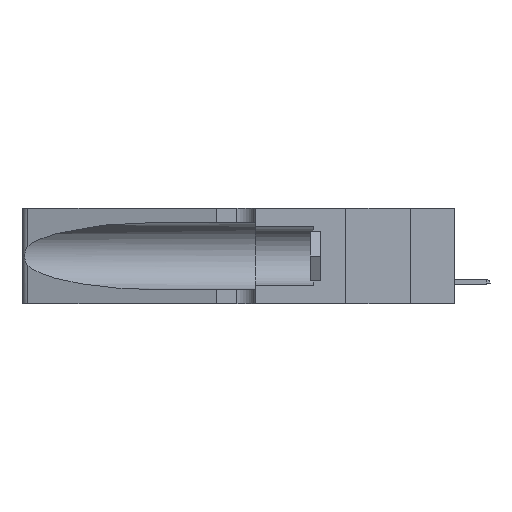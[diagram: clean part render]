
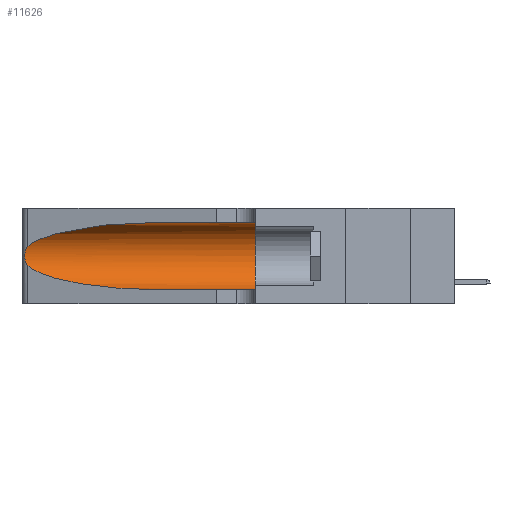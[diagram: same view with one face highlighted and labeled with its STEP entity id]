
A CAD part, left-side view. The second image highlights one B-rep face of the part: STEP entity #11626.
In plain terms, the highlighted cylindrical face has radius 3.308 mm (diameter 6.617 mm), a partial arc.
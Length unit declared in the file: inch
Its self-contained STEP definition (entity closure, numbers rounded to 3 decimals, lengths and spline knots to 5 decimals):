
#151 = VERTEX_POINT ( 'NONE', #3501 ) ;
#190 = DIRECTION ( 'NONE',  ( 0., -1., 0. ) ) ;
#1014 = CARTESIAN_POINT ( 'NONE',  ( 0.18966, 0.96281, 0.31525 ) ) ;
#1051 = CARTESIAN_POINT ( 'NONE',  ( 0.25555, 1.22993, 0.14849 ) ) ;
#1424 = CARTESIAN_POINT ( 'NONE',  ( 0.25787, 1.23484, 0.2124 ) ) ;
#2444 = CARTESIAN_POINT ( 'NONE',  ( 0.25487, 1.22718, 0.14631 ) ) ;
#2725 = VECTOR ( 'NONE', #190, 39.37008 ) ;
#3114 = CARTESIAN_POINT ( 'NONE',  ( 0.26075, 1.23896, 0.178 ) ) ;
#3232 = EDGE_CURVE ( 'NONE', #11113, #3688, #13673, .T. ) ;
#3237 = CARTESIAN_POINT ( 'NONE',  ( 0.26017, 1.23833, 0.17102 ) ) ;
#3501 = CARTESIAN_POINT ( 'NONE',  ( 0.1305, 0.72297, 0.31525 ) ) ;
#3611 = CARTESIAN_POINT ( 'NONE',  ( 0.25487, 1.22718, 0.22369 ) ) ;
#3688 = VERTEX_POINT ( 'NONE', #20393 ) ;
#4425 = B_SPLINE_CURVE_WITH_KNOTS ( 'NONE', 3,
 ( #3611, #5035, #24496, #1424, #21156, #20654, #14872, #3114, #3237, #16923, #13206, #11416, #1051, #5421 ),
 .UNSPECIFIED., .F., .F.,
 ( 4, 2, 2, 2, 2, 2, 4 ),
 ( 0., 0.00027, 0.00053, 0.00107, 0.0016, 0.00187, 0.00214 ),
 .UNSPECIFIED. ) ;
#4504 = CARTESIAN_POINT ( 'NONE',  ( 0.25487, 1.22718, 0.22369 ) ) ;
#4877 = CARTESIAN_POINT ( 'NONE',  ( 0.1305, 0.35, 0.31525 ) ) ;
#5028 = EDGE_CURVE ( 'NONE', #7660, #12169, #4425, .T. ) ;
#5035 = CARTESIAN_POINT ( 'NONE',  ( 0.25555, 1.22994, 0.2215 ) ) ;
#5104 = EDGE_CURVE ( 'NONE', #151, #11113, #6177, .T. ) ;
#5421 = CARTESIAN_POINT ( 'NONE',  ( 0.25487, 1.22718, 0.14631 ) ) ;
#5674 = ORIENTED_EDGE ( 'NONE', *, *, #12125, .T. ) ;
#6177 = LINE ( 'NONE', #19471, #2725 ) ;
#6364 = DIRECTION ( 'NONE',  ( 0., 0., 1. ) ) ;
#6689 =( BOUNDED_CURVE ( )  B_SPLINE_CURVE ( 3, ( #16148, #14227, #23962, #22038 ),
 .UNSPECIFIED., .F., .F. ) 
 B_SPLINE_CURVE_WITH_KNOTS ( ( 4, 4 ),
 ( 3.44316, 4.71239 ),
 .UNSPECIFIED. ) 
 CURVE ( )  GEOMETRIC_REPRESENTATION_ITEM ( )  RATIONAL_B_SPLINE_CURVE ( ( 1., 0.87, 0.87, 1. ) ) 
 REPRESENTATION_ITEM ( '' )  );
#6929 = CARTESIAN_POINT ( 'NONE',  ( 0.1305, 0.72297, 0.31525 ) ) ;
#7660 = VERTEX_POINT ( 'NONE', #21090 ) ;
#7761 = CARTESIAN_POINT ( 'NONE',  ( 0.1305, 0.72297, 0.05475 ) ) ;
#8336 =( BOUNDED_CURVE ( )  B_SPLINE_CURVE ( 3, ( #6929, #1014, #8735, #4504 ),
 .UNSPECIFIED., .F., .T. ) 
 B_SPLINE_CURVE_WITH_KNOTS ( ( 4, 4 ),
 ( 1.5708, 2.84003 ),
 .UNSPECIFIED. ) 
 CURVE ( )  GEOMETRIC_REPRESENTATION_ITEM ( )  RATIONAL_B_SPLINE_CURVE ( ( 1., 0.87, 0.87, 1. ) ) 
 REPRESENTATION_ITEM ( '' )  );
#8735 = CARTESIAN_POINT ( 'NONE',  ( 0.2373, 1.15595, 0.28018 ) ) ;
#8787 = EDGE_CURVE ( 'NONE', #151, #7660, #8336, .T. ) ;
#10125 = DIRECTION ( 'NONE',  ( 0., -1., 0. ) ) ;
#10908 = EDGE_LOOP ( 'NONE', ( #15554, #25316, #5674, #13364, #15202, #18108 ) ) ;
#11113 = VERTEX_POINT ( 'NONE', #4877 ) ;
#11416 = CARTESIAN_POINT ( 'NONE',  ( 0.25639, 1.23186, 0.15144 ) ) ;
#11603 = CYLINDRICAL_SURFACE ( 'NONE', #22852, 0.13025 ) ;
#11626 = ADVANCED_FACE ( 'NONE', ( #15311 ), #11603, .F. ) ;
#12125 = EDGE_CURVE ( 'NONE', #12169, #19069, #6689, .T. ) ;
#12169 = VERTEX_POINT ( 'NONE', #2444 ) ;
#13206 = CARTESIAN_POINT ( 'NONE',  ( 0.25789, 1.23486, 0.15765 ) ) ;
#13364 = ORIENTED_EDGE ( 'NONE', *, *, #24914, .T. ) ;
#13673 = CIRCLE ( 'NONE', #21056, 0.13025 ) ;
#13943 = CARTESIAN_POINT ( 'NONE',  ( 0.1305, 1.61858, 0.05475 ) ) ;
#14161 = CARTESIAN_POINT ( 'NONE',  ( 0.1305, 0.35, 0.185 ) ) ;
#14227 = CARTESIAN_POINT ( 'NONE',  ( 0.2373, 1.15595, 0.08982 ) ) ;
#14276 = DIRECTION ( 'NONE',  ( 0., 1., 0. ) ) ;
#14872 = CARTESIAN_POINT ( 'NONE',  ( 0.26075, 1.23896, 0.19203 ) ) ;
#15202 = ORIENTED_EDGE ( 'NONE', *, *, #3232, .F. ) ;
#15311 = FACE_OUTER_BOUND ( 'NONE', #10908, .T. ) ;
#15554 = ORIENTED_EDGE ( 'NONE', *, *, #8787, .T. ) ;
#16148 = CARTESIAN_POINT ( 'NONE',  ( 0.25487, 1.22718, 0.14631 ) ) ;
#16923 = CARTESIAN_POINT ( 'NONE',  ( 0.25856, 1.23593, 0.16098 ) ) ;
#17348 = CARTESIAN_POINT ( 'NONE',  ( 0.1305, 1.61858, 0.185 ) ) ;
#18108 = ORIENTED_EDGE ( 'NONE', *, *, #5104, .F. ) ;
#19069 = VERTEX_POINT ( 'NONE', #7761 ) ;
#19471 = CARTESIAN_POINT ( 'NONE',  ( 0.1305, 1.61858, 0.31525 ) ) ;
#19574 = LINE ( 'NONE', #13943, #23394 ) ;
#20393 = CARTESIAN_POINT ( 'NONE',  ( 0.1305, 0.35, 0.05475 ) ) ;
#20654 = CARTESIAN_POINT ( 'NONE',  ( 0.26018, 1.23835, 0.19895 ) ) ;
#21056 = AXIS2_PLACEMENT_3D ( 'NONE', #14161, #14276, #6364 ) ;
#21090 = CARTESIAN_POINT ( 'NONE',  ( 0.25487, 1.22718, 0.22369 ) ) ;
#21156 = CARTESIAN_POINT ( 'NONE',  ( 0.25854, 1.2359, 0.20912 ) ) ;
#22038 = CARTESIAN_POINT ( 'NONE',  ( 0.1305, 0.72297, 0.05475 ) ) ;
#22852 = AXIS2_PLACEMENT_3D ( 'NONE', #17348, #23002, #22880 ) ;
#22880 = DIRECTION ( 'NONE',  ( 0., 0., -1. ) ) ;
#23002 = DIRECTION ( 'NONE',  ( 0., -1., 0. ) ) ;
#23394 = VECTOR ( 'NONE', #10125, 39.37008 ) ;
#23962 = CARTESIAN_POINT ( 'NONE',  ( 0.18966, 0.96281, 0.05475 ) ) ;
#24496 = CARTESIAN_POINT ( 'NONE',  ( 0.25639, 1.23184, 0.21858 ) ) ;
#24914 = EDGE_CURVE ( 'NONE', #19069, #3688, #19574, .T. ) ;
#25316 = ORIENTED_EDGE ( 'NONE', *, *, #5028, .T. ) ;
